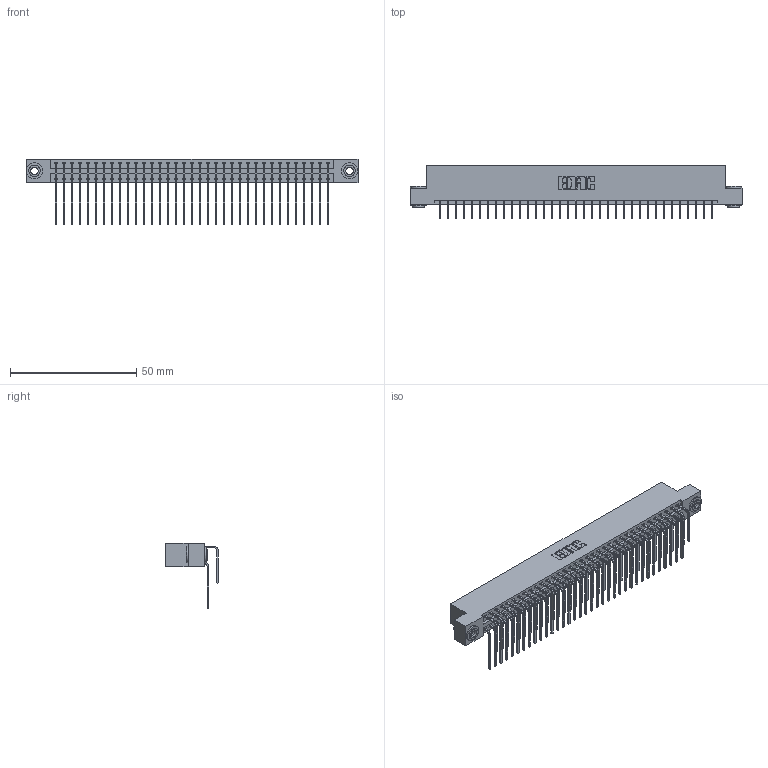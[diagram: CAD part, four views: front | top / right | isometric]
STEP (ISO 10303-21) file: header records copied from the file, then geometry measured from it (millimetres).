
FILE_DESCRIPTION (( 'STEP AP203' ), '1' );
FILE_NAME ('346-070-559-203.STEP', '2022-05-24T22:28:13', ( '' ), ( '' ), 'SwSTEP 2.0', 'SolidWorks 2020', '' );
FILE_SCHEMA (( 'CONFIG_CONTROL_DESIGN' ));
Length unit declared in the file: inch
Products named in the file (5): 345-292-001_558 559 Tail - 1; 346 Part_Flush Mounting Lugs - 0.156 Dia-TH; 345-250-002_345-250-002-102; 345-292-001_559 Tail - 2; 346-070-559-203
Assembly tree (73 placements, depth 2):
  346-070-559-203
    346 Part_Flush Mounting Lugs - 0.156 Dia-TH
    345-292-001_558 559 Tail - 1  x35
    345-292-001_559 Tail - 2  x35
    345-250-002_345-250-002-102  x2
Bounding box: 131.7 x 20.89 x 26.16 mm (x, y, z)
Volume: 13193 mm3; surface area: 20210.6 mm2
Topology: 73 solids, 73 shells, 3954 faces, 11711 edges, 7710 vertices
Faces by surface type: plane 2690, cylinder 1256, cone 8
Entity records: 26634 total; most frequent: CARTESIAN_POINT 4432, ORIENTED_EDGE 4306, DIRECTION 3959, EDGE_CURVE 2153, VECTOR 1817, LINE 1817, VERTEX_POINT 1430, AXIS2_PLACEMENT_3D 1071
